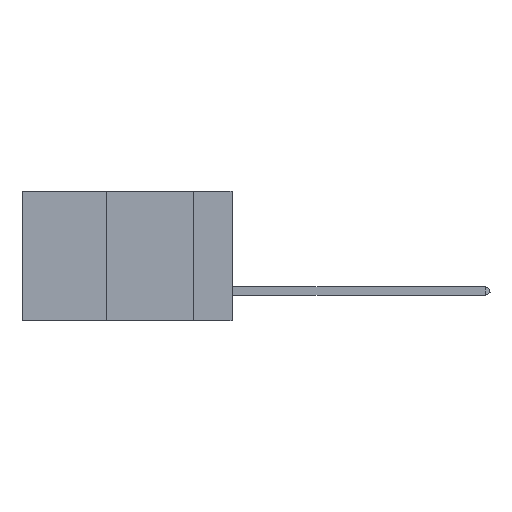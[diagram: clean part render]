
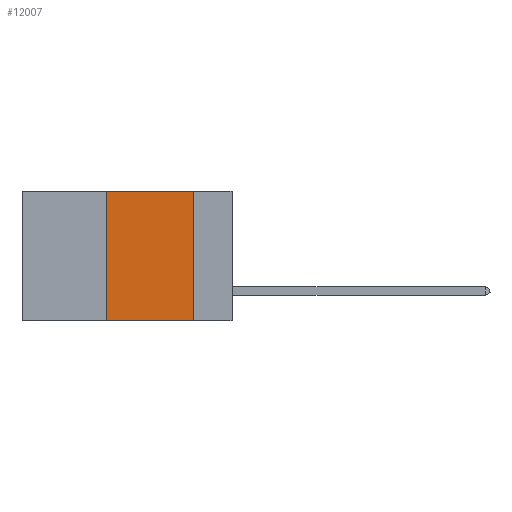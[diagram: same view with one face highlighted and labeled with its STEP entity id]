
A CAD part, left-side view. The second image highlights one B-rep face of the part: STEP entity #12007.
In plain terms, the highlighted planar face has unit normal (-1, 0, 0).
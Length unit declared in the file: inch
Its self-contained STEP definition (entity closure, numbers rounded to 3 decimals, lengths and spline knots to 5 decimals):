
#816 = EDGE_CURVE ( 'NONE', #38212, #29780, #6893, .T. ) ;
#5966 = ORIENTED_EDGE ( 'NONE', *, *, #9998, .F. ) ;
#6893 = LINE ( 'NONE', #44332, #18262 ) ;
#7473 = EDGE_LOOP ( 'NONE', ( #18300, #20402, #5966, #47856 ) ) ;
#8407 = DIRECTION ( 'NONE',  ( 0., 0., -1. ) ) ;
#9998 = EDGE_CURVE ( 'NONE', #38212, #39583, #21785, .T. ) ;
#10488 = DIRECTION ( 'NONE',  ( 0., -1., 0. ) ) ;
#12007 = ADVANCED_FACE ( 'NONE', ( #36185 ), #32304, .F. ) ;
#12620 = VERTEX_POINT ( 'NONE', #28830 ) ;
#13474 = CARTESIAN_POINT ( 'NONE',  ( 0., 0.6, 0. ) ) ;
#14757 = DIRECTION ( 'NONE',  ( 0., 0., -1. ) ) ;
#16146 = VECTOR ( 'NONE', #16917, 39.37008 ) ;
#16650 = AXIS2_PLACEMENT_3D ( 'NONE', #13474, #46295, #8407 ) ;
#16917 = DIRECTION ( 'NONE',  ( 0., -1., 0. ) ) ;
#18262 = VECTOR ( 'NONE', #10488, 39.37008 ) ;
#18300 = ORIENTED_EDGE ( 'NONE', *, *, #40893, .F. ) ;
#18647 = EDGE_CURVE ( 'NONE', #39583, #12620, #45551, .T. ) ;
#20402 = ORIENTED_EDGE ( 'NONE', *, *, #18647, .F. ) ;
#21785 = LINE ( 'NONE', #38259, #25404 ) ;
#24926 = VECTOR ( 'NONE', #14757, 39.37008 ) ;
#25404 = VECTOR ( 'NONE', #43583, 39.37008 ) ;
#28514 = CARTESIAN_POINT ( 'NONE',  ( 0., 0.11, -0.37 ) ) ;
#28830 = CARTESIAN_POINT ( 'NONE',  ( 0., 0.11, 0. ) ) ;
#29780 = VERTEX_POINT ( 'NONE', #28514 ) ;
#30295 = CARTESIAN_POINT ( 'NONE',  ( 0., 0.11, 0. ) ) ;
#30359 = CARTESIAN_POINT ( 'NONE',  ( 0., 0.36, -0.37 ) ) ;
#31937 = CARTESIAN_POINT ( 'NONE',  ( 0., 0.36, 0. ) ) ;
#32304 = PLANE ( 'NONE',  #16650 ) ;
#35167 = LINE ( 'NONE', #30295, #24926 ) ;
#36185 = FACE_OUTER_BOUND ( 'NONE', #7473, .T. ) ;
#38212 = VERTEX_POINT ( 'NONE', #30359 ) ;
#38259 = CARTESIAN_POINT ( 'NONE',  ( 0., 0.36, 0. ) ) ;
#38542 = CARTESIAN_POINT ( 'NONE',  ( 0., 0.6, 0. ) ) ;
#39583 = VERTEX_POINT ( 'NONE', #31937 ) ;
#40893 = EDGE_CURVE ( 'NONE', #12620, #29780, #35167, .T. ) ;
#43583 = DIRECTION ( 'NONE',  ( 0., 0., 1. ) ) ;
#44332 = CARTESIAN_POINT ( 'NONE',  ( 0., 0.6, -0.37 ) ) ;
#45551 = LINE ( 'NONE', #38542, #16146 ) ;
#46295 = DIRECTION ( 'NONE',  ( 1., 0., 0. ) ) ;
#47856 = ORIENTED_EDGE ( 'NONE', *, *, #816, .T. ) ;
